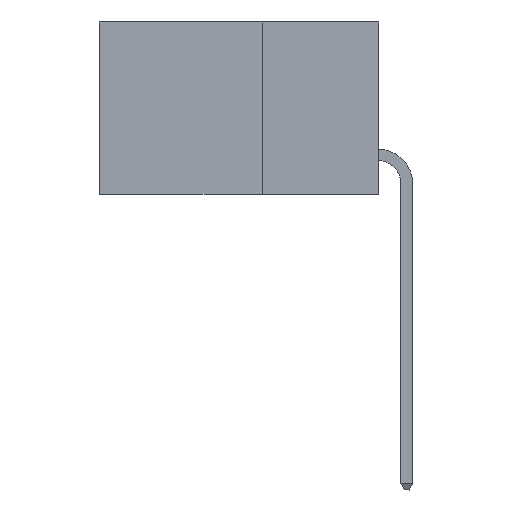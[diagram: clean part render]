
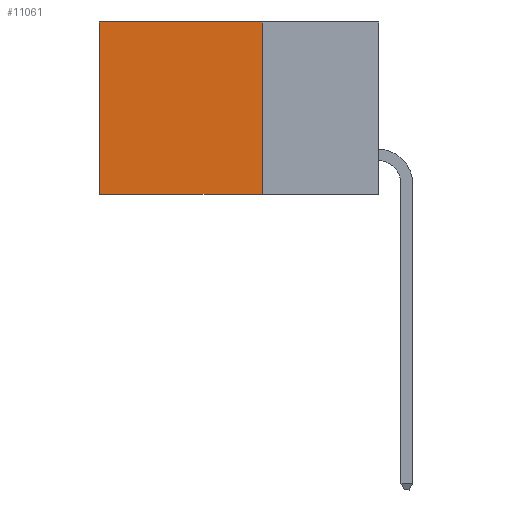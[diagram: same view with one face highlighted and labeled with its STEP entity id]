
A CAD part, left-side view. The second image highlights one B-rep face of the part: STEP entity #11061.
In plain terms, the highlighted planar face has unit normal (-1, 0, 0).
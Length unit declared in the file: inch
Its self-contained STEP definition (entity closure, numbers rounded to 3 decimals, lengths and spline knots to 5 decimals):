
#79 = LINE ( 'NONE', #10460, #5929 ) ;
#597 = VERTEX_POINT ( 'NONE', #7773 ) ;
#714 = LINE ( 'NONE', #11424, #12298 ) ;
#1080 = LINE ( 'NONE', #2345, #6900 ) ;
#1126 = CARTESIAN_POINT ( 'NONE',  ( 0.298, 0.25, 0. ) ) ;
#1624 = DIRECTION ( 'NONE',  ( 0., 1., 0. ) ) ;
#2345 = CARTESIAN_POINT ( 'NONE',  ( 0.298, 0.25, -0.37 ) ) ;
#2444 = VERTEX_POINT ( 'NONE', #11428 ) ;
#2921 = CARTESIAN_POINT ( 'NONE',  ( 0.298, 0.6, -0.37 ) ) ;
#3368 = DIRECTION ( 'NONE',  ( 0., 0., -1. ) ) ;
#3771 = LINE ( 'NONE', #7328, #9192 ) ;
#5066 = DIRECTION ( 'NONE',  ( 0., 0., -1. ) ) ;
#5205 = ORIENTED_EDGE ( 'NONE', *, *, #5879, .T. ) ;
#5879 = EDGE_CURVE ( 'NONE', #597, #6322, #714, .T. ) ;
#5929 = VECTOR ( 'NONE', #5066, 39.37008 ) ;
#6322 = VERTEX_POINT ( 'NONE', #6801 ) ;
#6801 = CARTESIAN_POINT ( 'NONE',  ( 0.298, 0.6, 0. ) ) ;
#6900 = VECTOR ( 'NONE', #12115, 39.37008 ) ;
#7196 = FACE_OUTER_BOUND ( 'NONE', #12669, .T. ) ;
#7328 = CARTESIAN_POINT ( 'NONE',  ( 0.298, 0.6, 0. ) ) ;
#7437 = ORIENTED_EDGE ( 'NONE', *, *, #9894, .F. ) ;
#7771 = ORIENTED_EDGE ( 'NONE', *, *, #13750, .T. ) ;
#7773 = CARTESIAN_POINT ( 'NONE',  ( 0.298, 0.25, 0. ) ) ;
#8237 = EDGE_CURVE ( 'NONE', #597, #2444, #79, .T. ) ;
#8423 = DIRECTION ( 'NONE',  ( 0., 0., -1. ) ) ;
#9192 = VECTOR ( 'NONE', #8423, 39.37008 ) ;
#9883 = DIRECTION ( 'NONE',  ( 1., 0., 0. ) ) ;
#9894 = EDGE_CURVE ( 'NONE', #2444, #11949, #1080, .T. ) ;
#10460 = CARTESIAN_POINT ( 'NONE',  ( 0.298, 0.25, 0. ) ) ;
#11061 = ADVANCED_FACE ( 'NONE', ( #7196 ), #13066, .F. ) ;
#11107 = AXIS2_PLACEMENT_3D ( 'NONE', #1126, #9883, #3368 ) ;
#11277 = ORIENTED_EDGE ( 'NONE', *, *, #8237, .F. ) ;
#11424 = CARTESIAN_POINT ( 'NONE',  ( 0.298, 0.25, 0. ) ) ;
#11428 = CARTESIAN_POINT ( 'NONE',  ( 0.298, 0.25, -0.37 ) ) ;
#11949 = VERTEX_POINT ( 'NONE', #2921 ) ;
#12115 = DIRECTION ( 'NONE',  ( 0., 1., 0. ) ) ;
#12298 = VECTOR ( 'NONE', #1624, 39.37008 ) ;
#12669 = EDGE_LOOP ( 'NONE', ( #7771, #7437, #11277, #5205 ) ) ;
#13066 = PLANE ( 'NONE',  #11107 ) ;
#13750 = EDGE_CURVE ( 'NONE', #6322, #11949, #3771, .T. ) ;
